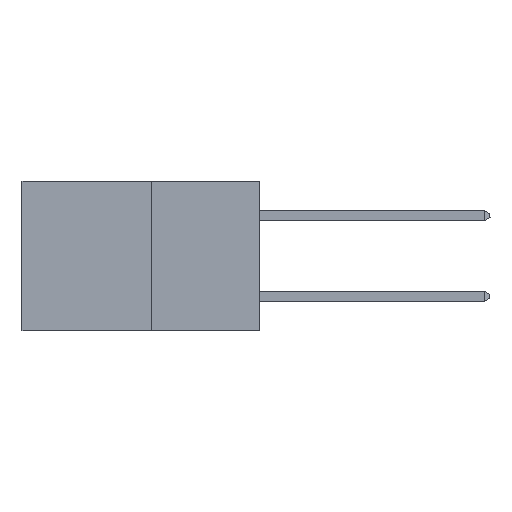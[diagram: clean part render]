
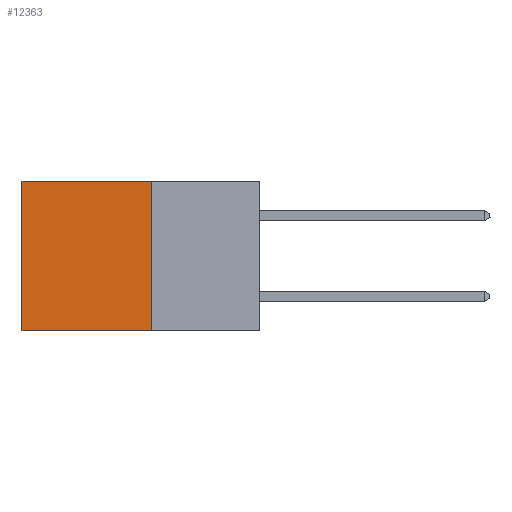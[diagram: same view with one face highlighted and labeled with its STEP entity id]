
A CAD part, left-side view. The second image highlights one B-rep face of the part: STEP entity #12363.
In plain terms, the highlighted planar face has unit normal (-1, 0, 0).
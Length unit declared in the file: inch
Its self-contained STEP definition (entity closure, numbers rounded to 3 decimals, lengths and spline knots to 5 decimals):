
#188 = CARTESIAN_POINT ( 'NONE',  ( 0.277, 0.27, -0.37 ) ) ;
#728 = DIRECTION ( 'NONE',  ( 0., 1., 0. ) ) ;
#1010 = CARTESIAN_POINT ( 'NONE',  ( 0.277, 0.27, 0. ) ) ;
#2695 = ORIENTED_EDGE ( 'NONE', *, *, #12854, .F. ) ;
#2703 = DIRECTION ( 'NONE',  ( 0., 1., 0. ) ) ;
#3178 = EDGE_CURVE ( 'NONE', #15040, #14997, #12751, .T. ) ;
#3706 = DIRECTION ( 'NONE',  ( 0., 0., -1. ) ) ;
#3950 = EDGE_CURVE ( 'NONE', #7399, #14997, #7897, .T. ) ;
#3957 = VECTOR ( 'NONE', #3706, 39.37008 ) ;
#4277 = VECTOR ( 'NONE', #5611, 39.37008 ) ;
#4824 = CARTESIAN_POINT ( 'NONE',  ( 0.277, 0.59, -0.37 ) ) ;
#4980 = AXIS2_PLACEMENT_3D ( 'NONE', #6143, #17402, #7815 ) ;
#5152 = ORIENTED_EDGE ( 'NONE', *, *, #3178, .T. ) ;
#5398 = VECTOR ( 'NONE', #2703, 39.37008 ) ;
#5611 = DIRECTION ( 'NONE',  ( 0., 0., -1. ) ) ;
#5785 = EDGE_LOOP ( 'NONE', ( #5152, #10687, #2695, #18363 ) ) ;
#6136 = VERTEX_POINT ( 'NONE', #8307 ) ;
#6143 = CARTESIAN_POINT ( 'NONE',  ( 0.277, 0.27, -0.37 ) ) ;
#7205 = EDGE_CURVE ( 'NONE', #6136, #15040, #14141, .T. ) ;
#7399 = VERTEX_POINT ( 'NONE', #13108 ) ;
#7815 = DIRECTION ( 'NONE',  ( 0., 0., -1. ) ) ;
#7897 = LINE ( 'NONE', #188, #19605 ) ;
#8221 = LINE ( 'NONE', #13797, #4277 ) ;
#8307 = CARTESIAN_POINT ( 'NONE',  ( 0.277, 0.27, 0. ) ) ;
#10687 = ORIENTED_EDGE ( 'NONE', *, *, #3950, .F. ) ;
#11045 = PLANE ( 'NONE',  #4980 ) ;
#12135 = CARTESIAN_POINT ( 'NONE',  ( 0.277, 0.59, -0.37 ) ) ;
#12363 = ADVANCED_FACE ( 'NONE', ( #13087 ), #11045, .F. ) ;
#12751 = LINE ( 'NONE', #4824, #3957 ) ;
#12854 = EDGE_CURVE ( 'NONE', #6136, #7399, #8221, .T. ) ;
#13087 = FACE_OUTER_BOUND ( 'NONE', #5785, .T. ) ;
#13108 = CARTESIAN_POINT ( 'NONE',  ( 0.277, 0.27, -0.37 ) ) ;
#13797 = CARTESIAN_POINT ( 'NONE',  ( 0.277, 0.27, -0.37 ) ) ;
#14141 = LINE ( 'NONE', #1010, #5398 ) ;
#14997 = VERTEX_POINT ( 'NONE', #12135 ) ;
#15040 = VERTEX_POINT ( 'NONE', #18521 ) ;
#17402 = DIRECTION ( 'NONE',  ( 1., 0., 0. ) ) ;
#18363 = ORIENTED_EDGE ( 'NONE', *, *, #7205, .T. ) ;
#18521 = CARTESIAN_POINT ( 'NONE',  ( 0.277, 0.59, 0. ) ) ;
#19605 = VECTOR ( 'NONE', #728, 39.37008 ) ;
